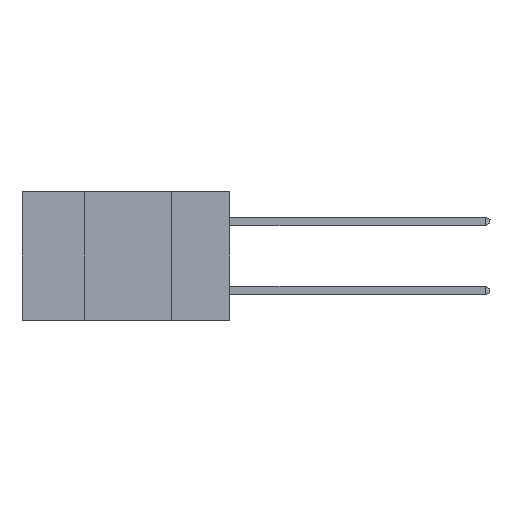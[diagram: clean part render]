
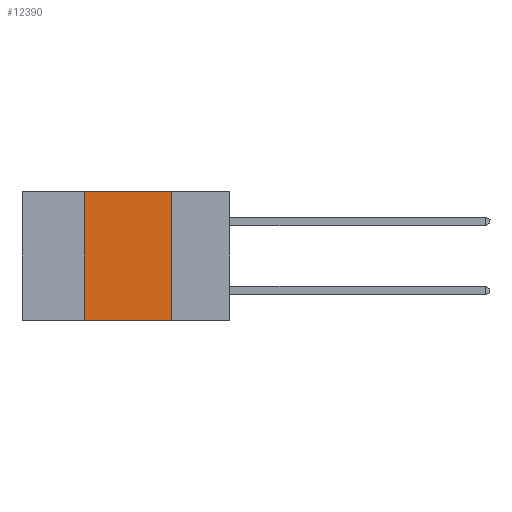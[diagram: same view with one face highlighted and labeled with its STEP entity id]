
A CAD part, left-side view. The second image highlights one B-rep face of the part: STEP entity #12390.
In plain terms, the highlighted planar face has unit normal (-1, 0, 0).
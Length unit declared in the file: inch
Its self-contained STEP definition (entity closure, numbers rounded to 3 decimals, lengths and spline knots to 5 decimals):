
#111 = CARTESIAN_POINT ( 'NONE',  ( 0., 0.42, -0.37 ) ) ;
#281 = CARTESIAN_POINT ( 'NONE',  ( 0., 0.6, 0. ) ) ;
#518 = CARTESIAN_POINT ( 'NONE',  ( 0., 0.42, -0.37 ) ) ;
#2054 = DIRECTION ( 'NONE',  ( 0., -1., 0. ) ) ;
#2166 = ORIENTED_EDGE ( 'NONE', *, *, #12899, .T. ) ;
#2344 = CARTESIAN_POINT ( 'NONE',  ( 0., 0.42, 0. ) ) ;
#3240 = LINE ( 'NONE', #111, #10383 ) ;
#3303 = PLANE ( 'NONE',  #10891 ) ;
#3468 = CARTESIAN_POINT ( 'NONE',  ( 0., 0.6, 0. ) ) ;
#3579 = DIRECTION ( 'NONE',  ( 0., -1., 0. ) ) ;
#4519 = CARTESIAN_POINT ( 'NONE',  ( 0., 0.17, -0.37 ) ) ;
#5109 = ORIENTED_EDGE ( 'NONE', *, *, #18989, .F. ) ;
#5748 = VECTOR ( 'NONE', #3579, 39.37008 ) ;
#6148 = ORIENTED_EDGE ( 'NONE', *, *, #7039, .F. ) ;
#6984 = VERTEX_POINT ( 'NONE', #14855 ) ;
#7039 = EDGE_CURVE ( 'NONE', #9342, #6984, #18375, .T. ) ;
#9342 = VERTEX_POINT ( 'NONE', #12360 ) ;
#9354 = CARTESIAN_POINT ( 'NONE',  ( 0., 0.6, -0.37 ) ) ;
#10383 = VECTOR ( 'NONE', #12536, 39.37008 ) ;
#10575 = VERTEX_POINT ( 'NONE', #518 ) ;
#10891 = AXIS2_PLACEMENT_3D ( 'NONE', #281, #11093, #15950 ) ;
#11093 = DIRECTION ( 'NONE',  ( 1., 0., 0. ) ) ;
#12009 = DIRECTION ( 'NONE',  ( 0., 0., -1. ) ) ;
#12360 = CARTESIAN_POINT ( 'NONE',  ( 0., 0.17, 0. ) ) ;
#12390 = ADVANCED_FACE ( 'NONE', ( #12500 ), #3303, .F. ) ;
#12500 = FACE_OUTER_BOUND ( 'NONE', #18976, .T. ) ;
#12536 = DIRECTION ( 'NONE',  ( 0., 0., 1. ) ) ;
#12899 = EDGE_CURVE ( 'NONE', #10575, #6984, #15514, .T. ) ;
#13435 = VERTEX_POINT ( 'NONE', #2344 ) ;
#13698 = ORIENTED_EDGE ( 'NONE', *, *, #14045, .F. ) ;
#14045 = EDGE_CURVE ( 'NONE', #13435, #9342, #14496, .T. ) ;
#14496 = LINE ( 'NONE', #3468, #14515 ) ;
#14515 = VECTOR ( 'NONE', #2054, 39.37008 ) ;
#14855 = CARTESIAN_POINT ( 'NONE',  ( 0., 0.17, -0.37 ) ) ;
#15514 = LINE ( 'NONE', #9354, #5748 ) ;
#15621 = VECTOR ( 'NONE', #12009, 39.37008 ) ;
#15950 = DIRECTION ( 'NONE',  ( 0., 0., -1. ) ) ;
#18375 = LINE ( 'NONE', #4519, #15621 ) ;
#18976 = EDGE_LOOP ( 'NONE', ( #6148, #13698, #5109, #2166 ) ) ;
#18989 = EDGE_CURVE ( 'NONE', #10575, #13435, #3240, .T. ) ;
